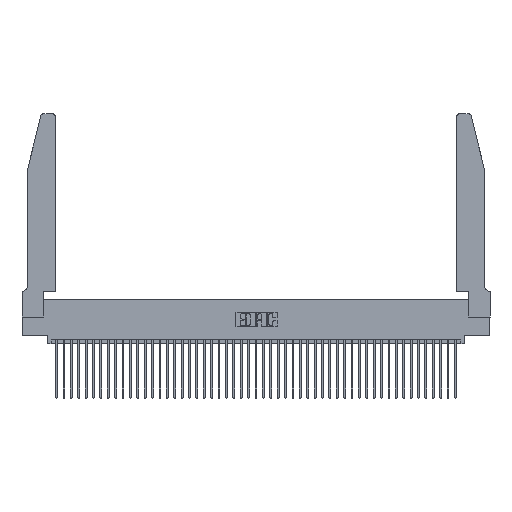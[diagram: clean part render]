
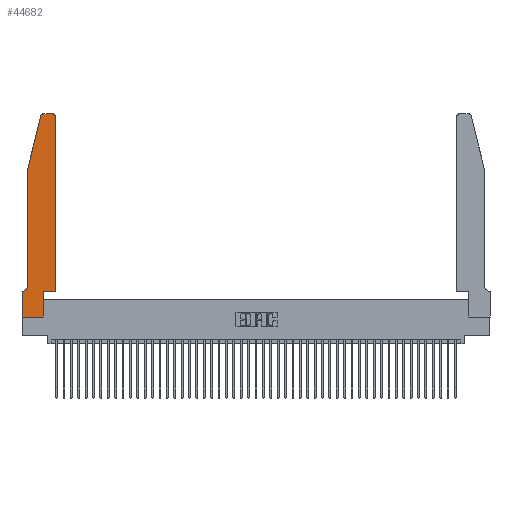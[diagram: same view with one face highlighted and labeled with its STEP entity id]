
A CAD part, top view. The second image highlights one B-rep face of the part: STEP entity #44682.
In plain terms, the highlighted planar face has unit normal (0, 0, 1).
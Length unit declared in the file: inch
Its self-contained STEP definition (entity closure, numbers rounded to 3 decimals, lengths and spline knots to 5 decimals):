
#16 = ORIENTED_EDGE ( 'NONE', *, *, #21388, .T. ) ;
#149 = LINE ( 'NONE', #30928, #18245 ) ;
#684 = CARTESIAN_POINT ( 'NONE',  ( 0.4505, 0.35, 0.37 ) ) ;
#805 = AXIS2_PLACEMENT_3D ( 'NONE', #18015, #10960, #35905 ) ;
#1309 = LINE ( 'NONE', #1370, #38315 ) ;
#1370 = CARTESIAN_POINT ( 'NONE',  ( 0.2605, 2.75, 0.37 ) ) ;
#2223 = AXIS2_PLACEMENT_3D ( 'NONE', #39463, #18166, #43007 ) ;
#2297 = VERTEX_POINT ( 'NONE', #15791 ) ;
#2465 = CIRCLE ( 'NONE', #2223, 0.07 ) ;
#3009 = EDGE_CURVE ( 'NONE', #27597, #22937, #2465, .T. ) ;
#3297 = LINE ( 'NONE', #17259, #39072 ) ;
#4374 = DIRECTION ( 'NONE',  ( 0., 1., 0. ) ) ;
#4896 = CARTESIAN_POINT ( 'NONE',  ( 0., 0., 0.37 ) ) ;
#5547 = EDGE_CURVE ( 'NONE', #22937, #29494, #10782, .T. ) ;
#6066 = VERTEX_POINT ( 'NONE', #27521 ) ;
#6424 = DIRECTION ( 'NONE',  ( 0., -1., 0. ) ) ;
#6490 = FACE_OUTER_BOUND ( 'NONE', #12621, .T. ) ;
#6796 = LINE ( 'NONE', #39732, #33052 ) ;
#7085 = CARTESIAN_POINT ( 'NONE',  ( 0.0755, 0.35, 0.37 ) ) ;
#7355 = PLANE ( 'NONE',  #805 ) ;
#8350 = EDGE_CURVE ( 'NONE', #32677, #2297, #6796, .T. ) ;
#8687 = ORIENTED_EDGE ( 'NONE', *, *, #19888, .T. ) ;
#9367 = EDGE_CURVE ( 'NONE', #29494, #32677, #3297, .T. ) ;
#9805 = DIRECTION ( 'NONE',  ( 0., -1., 0. ) ) ;
#10037 = CIRCLE ( 'NONE', #15278, 0.03 ) ;
#10703 = CIRCLE ( 'NONE', #32699, 0.03 ) ;
#10782 = LINE ( 'NONE', #7085, #14848 ) ;
#10960 = DIRECTION ( 'NONE',  ( 0., 0., 1. ) ) ;
#11239 = DIRECTION ( 'NONE',  ( 1., 0., 0. ) ) ;
#11328 = VECTOR ( 'NONE', #31718, 39.37008 ) ;
#12066 = VERTEX_POINT ( 'NONE', #38610 ) ;
#12235 = VECTOR ( 'NONE', #4374, 39.37008 ) ;
#12621 = EDGE_LOOP ( 'NONE', ( #8687, #13980, #33201, #16, #32901, #36336, #12681, #20917, #43724, #24251, #34559, #18577 ) ) ;
#12681 = ORIENTED_EDGE ( 'NONE', *, *, #9367, .T. ) ;
#13108 = CARTESIAN_POINT ( 'NONE',  ( 0.284, 2.72, 0.37 ) ) ;
#13363 = LINE ( 'NONE', #684, #12235 ) ;
#13980 = ORIENTED_EDGE ( 'NONE', *, *, #18028, .T. ) ;
#14231 = CARTESIAN_POINT ( 'NONE',  ( 0.4505, 0.35, 0.37 ) ) ;
#14486 = VERTEX_POINT ( 'NONE', #37133 ) ;
#14848 = VECTOR ( 'NONE', #28519, 39.37008 ) ;
#15278 = AXIS2_PLACEMENT_3D ( 'NONE', #13108, #38043, #16723 ) ;
#15791 = CARTESIAN_POINT ( 'NONE',  ( 0.2865, 0., 0.37 ) ) ;
#16213 = EDGE_CURVE ( 'NONE', #14486, #38740, #39747, .T. ) ;
#16455 = CARTESIAN_POINT ( 'NONE',  ( 0.4205, 2.72, 0.37 ) ) ;
#16723 = DIRECTION ( 'NONE',  ( 1., 0., 0. ) ) ;
#17259 = CARTESIAN_POINT ( 'NONE',  ( 0., 0., 0.37 ) ) ;
#18015 = CARTESIAN_POINT ( 'NONE',  ( 0., 0.35, 0.37 ) ) ;
#18028 = EDGE_CURVE ( 'NONE', #12066, #14486, #10037, .T. ) ;
#18166 = DIRECTION ( 'NONE',  ( 0., 0., -1. ) ) ;
#18221 = VERTEX_POINT ( 'NONE', #35213 ) ;
#18245 = VECTOR ( 'NONE', #27329, 39.37008 ) ;
#18355 = CARTESIAN_POINT ( 'NONE',  ( 0.4505, 0.35, 0.37 ) ) ;
#18375 = CARTESIAN_POINT ( 'NONE',  ( 0.2865, 0.35, 0.37 ) ) ;
#18443 = EDGE_CURVE ( 'NONE', #41422, #6066, #13363, .T. ) ;
#18577 = ORIENTED_EDGE ( 'NONE', *, *, #34171, .T. ) ;
#19000 = VECTOR ( 'NONE', #35583, 39.37008 ) ;
#19888 = EDGE_CURVE ( 'NONE', #18221, #12066, #1309, .T. ) ;
#20023 = DIRECTION ( 'NONE',  ( 1., 0., 0. ) ) ;
#20917 = ORIENTED_EDGE ( 'NONE', *, *, #8350, .T. ) ;
#21388 = EDGE_CURVE ( 'NONE', #38740, #27597, #34218, .T. ) ;
#21708 = CARTESIAN_POINT ( 'NONE',  ( 0.0055, 0.35, 0.37 ) ) ;
#22690 = CARTESIAN_POINT ( 'NONE',  ( 0.0755, 2., 0.37 ) ) ;
#22937 = VERTEX_POINT ( 'NONE', #21708 ) ;
#23770 = EDGE_CURVE ( 'NONE', #24979, #41422, #26825, .T. ) ;
#24031 = CARTESIAN_POINT ( 'NONE',  ( 0.0755, 2., 0.37 ) ) ;
#24251 = ORIENTED_EDGE ( 'NONE', *, *, #23770, .T. ) ;
#24788 = VECTOR ( 'NONE', #9805, 39.37008 ) ;
#24979 = VERTEX_POINT ( 'NONE', #18375 ) ;
#26515 = DIRECTION ( 'NONE',  ( -1., 0., 0. ) ) ;
#26825 = LINE ( 'NONE', #14231, #19000 ) ;
#27329 = DIRECTION ( 'NONE',  ( 0., 1., 0. ) ) ;
#27521 = CARTESIAN_POINT ( 'NONE',  ( 0.4505, 2.72, 0.37 ) ) ;
#27597 = VERTEX_POINT ( 'NONE', #46321 ) ;
#28519 = DIRECTION ( 'NONE',  ( -1., 0., 0. ) ) ;
#29494 = VERTEX_POINT ( 'NONE', #34051 ) ;
#30928 = CARTESIAN_POINT ( 'NONE',  ( 0.2865, 0.35, 0.37 ) ) ;
#31718 = DIRECTION ( 'NONE',  ( -0.239, -0.971, 0. ) ) ;
#32677 = VERTEX_POINT ( 'NONE', #4896 ) ;
#32699 = AXIS2_PLACEMENT_3D ( 'NONE', #16455, #41305, #20023 ) ;
#32901 = ORIENTED_EDGE ( 'NONE', *, *, #3009, .T. ) ;
#33052 = VECTOR ( 'NONE', #11239, 39.37008 ) ;
#33201 = ORIENTED_EDGE ( 'NONE', *, *, #16213, .T. ) ;
#34051 = CARTESIAN_POINT ( 'NONE',  ( 0., 0.35, 0.37 ) ) ;
#34171 = EDGE_CURVE ( 'NONE', #6066, #18221, #10703, .T. ) ;
#34218 = LINE ( 'NONE', #24031, #24788 ) ;
#34559 = ORIENTED_EDGE ( 'NONE', *, *, #18443, .T. ) ;
#35213 = CARTESIAN_POINT ( 'NONE',  ( 0.4205, 2.75, 0.37 ) ) ;
#35271 = CARTESIAN_POINT ( 'NONE',  ( 0.0755, 2., 0.37 ) ) ;
#35583 = DIRECTION ( 'NONE',  ( 1., 0., 0. ) ) ;
#35905 = DIRECTION ( 'NONE',  ( 1., 0., 0. ) ) ;
#36336 = ORIENTED_EDGE ( 'NONE', *, *, #5547, .T. ) ;
#37133 = CARTESIAN_POINT ( 'NONE',  ( 0.25487, 2.72718, 0.37 ) ) ;
#38043 = DIRECTION ( 'NONE',  ( 0., 0., 1. ) ) ;
#38315 = VECTOR ( 'NONE', #26515, 39.37008 ) ;
#38610 = CARTESIAN_POINT ( 'NONE',  ( 0.284, 2.75, 0.37 ) ) ;
#38740 = VERTEX_POINT ( 'NONE', #22690 ) ;
#39072 = VECTOR ( 'NONE', #6424, 39.37008 ) ;
#39463 = CARTESIAN_POINT ( 'NONE',  ( 0.0055, 0.42, 0.37 ) ) ;
#39732 = CARTESIAN_POINT ( 'NONE',  ( 0., 0., 0.37 ) ) ;
#39747 = LINE ( 'NONE', #35271, #11328 ) ;
#41305 = DIRECTION ( 'NONE',  ( 0., 0., 1. ) ) ;
#41422 = VERTEX_POINT ( 'NONE', #18355 ) ;
#43007 = DIRECTION ( 'NONE',  ( -1., 0., 0. ) ) ;
#43724 = ORIENTED_EDGE ( 'NONE', *, *, #45061, .T. ) ;
#44682 = ADVANCED_FACE ( 'NONE', ( #6490 ), #7355, .T. ) ;
#45061 = EDGE_CURVE ( 'NONE', #2297, #24979, #149, .T. ) ;
#46321 = CARTESIAN_POINT ( 'NONE',  ( 0.0755, 0.42, 0.37 ) ) ;
